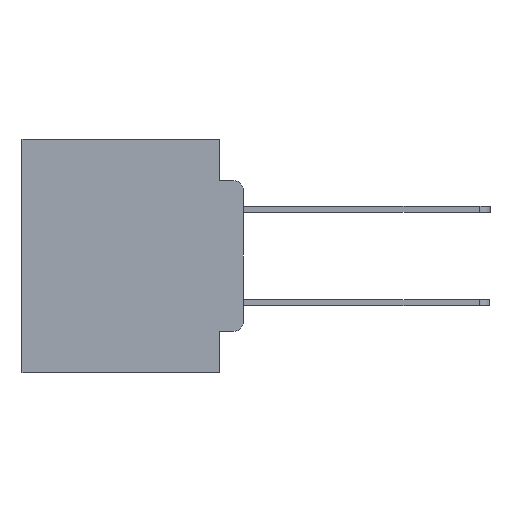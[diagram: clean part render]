
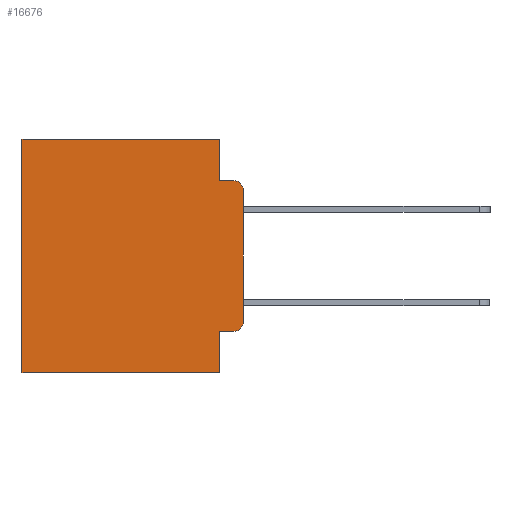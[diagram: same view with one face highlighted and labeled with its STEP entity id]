
A CAD part, left-side view. The second image highlights one B-rep face of the part: STEP entity #16676.
In plain terms, the highlighted planar face has unit normal (-1, 0, 0).
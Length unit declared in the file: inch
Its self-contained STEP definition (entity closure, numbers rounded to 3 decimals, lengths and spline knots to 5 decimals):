
#550 = LINE ( 'NONE', #1468, #6567 ) ;
#608 = VERTEX_POINT ( 'NONE', #22493 ) ;
#1370 = DIRECTION ( 'NONE',  ( 0., -1., 0. ) ) ;
#1468 = CARTESIAN_POINT ( 'NONE',  ( 0.298, 0.051, -0.0885 ) ) ;
#1498 = CARTESIAN_POINT ( 'NONE',  ( 0.298, 0., 0. ) ) ;
#1884 = ORIENTED_EDGE ( 'NONE', *, *, #14742, .F. ) ;
#2180 = VERTEX_POINT ( 'NONE', #12325 ) ;
#2238 = ORIENTED_EDGE ( 'NONE', *, *, #26624, .F. ) ;
#2448 = ORIENTED_EDGE ( 'NONE', *, *, #19890, .F. ) ;
#2474 = AXIS2_PLACEMENT_3D ( 'NONE', #1498, #10441, #24850 ) ;
#2882 = VECTOR ( 'NONE', #9533, 39.37008 ) ;
#3536 = CARTESIAN_POINT ( 'NONE',  ( 0.298, 0.051, -0.4115 ) ) ;
#3765 = CARTESIAN_POINT ( 'NONE',  ( 0.298, 0.473, 0. ) ) ;
#4331 = CARTESIAN_POINT ( 'NONE',  ( 0.298, 0.02, -0.1085 ) ) ;
#4355 = LINE ( 'NONE', #17075, #25990 ) ;
#4392 = CIRCLE ( 'NONE', #5933, 0.02 ) ;
#5150 = ORIENTED_EDGE ( 'NONE', *, *, #14354, .T. ) ;
#5281 = FACE_OUTER_BOUND ( 'NONE', #22569, .T. ) ;
#5768 = ORIENTED_EDGE ( 'NONE', *, *, #21215, .T. ) ;
#5933 = AXIS2_PLACEMENT_3D ( 'NONE', #4331, #19269, #6563 ) ;
#6232 = VERTEX_POINT ( 'NONE', #3765 ) ;
#6381 = DIRECTION ( 'NONE',  ( 0., 0., -1. ) ) ;
#6542 = VERTEX_POINT ( 'NONE', #9163 ) ;
#6563 = DIRECTION ( 'NONE',  ( 0., 0., -1. ) ) ;
#6567 = VECTOR ( 'NONE', #1370, 39.37008 ) ;
#6647 = EDGE_CURVE ( 'NONE', #6232, #12560, #23964, .T. ) ;
#7183 = EDGE_CURVE ( 'NONE', #18564, #608, #27380, .T. ) ;
#7649 = VERTEX_POINT ( 'NONE', #26843 ) ;
#8199 = VECTOR ( 'NONE', #15817, 39.37008 ) ;
#8276 = LINE ( 'NONE', #17052, #18820 ) ;
#9163 = CARTESIAN_POINT ( 'NONE',  ( 0.298, 0.051, -0.5 ) ) ;
#9533 = DIRECTION ( 'NONE',  ( 0., 0., -1. ) ) ;
#9902 = DIRECTION ( 'NONE',  ( -1., 0., 0. ) ) ;
#10441 = DIRECTION ( 'NONE',  ( 1., 0., 0. ) ) ;
#10773 = CARTESIAN_POINT ( 'NONE',  ( 0.298, 0.02, -0.0885 ) ) ;
#11007 = DIRECTION ( 'NONE',  ( 0., 0., -1. ) ) ;
#11294 = CARTESIAN_POINT ( 'NONE',  ( 0.298, 0.051, -0.4115 ) ) ;
#12325 = CARTESIAN_POINT ( 'NONE',  ( 0.298, 0.051, -0.0885 ) ) ;
#12560 = VERTEX_POINT ( 'NONE', #13832 ) ;
#13065 = VERTEX_POINT ( 'NONE', #17777 ) ;
#13832 = CARTESIAN_POINT ( 'NONE',  ( 0.298, 0.473, -0.5 ) ) ;
#13843 = CARTESIAN_POINT ( 'NONE',  ( 0.298, 0., 0. ) ) ;
#13853 = LINE ( 'NONE', #13843, #2882 ) ;
#14046 = ORIENTED_EDGE ( 'NONE', *, *, #19432, .F. ) ;
#14354 = EDGE_CURVE ( 'NONE', #13065, #6232, #14584, .T. ) ;
#14584 = LINE ( 'NONE', #25925, #8199 ) ;
#14742 = EDGE_CURVE ( 'NONE', #6542, #12560, #4355, .T. ) ;
#15424 = DIRECTION ( 'NONE',  ( 0., -1., 0. ) ) ;
#15817 = DIRECTION ( 'NONE',  ( 0., 1., 0. ) ) ;
#15904 = DIRECTION ( 'NONE',  ( 0., 0., -1. ) ) ;
#16362 = VERTEX_POINT ( 'NONE', #17791 ) ;
#16676 = ADVANCED_FACE ( 'NONE', ( #5281 ), #18743, .F. ) ;
#17052 = CARTESIAN_POINT ( 'NONE',  ( 0.298, 0.051, 0. ) ) ;
#17075 = CARTESIAN_POINT ( 'NONE',  ( 0.298, 0., -0.5 ) ) ;
#17703 = EDGE_CURVE ( 'NONE', #608, #16362, #23693, .T. ) ;
#17777 = CARTESIAN_POINT ( 'NONE',  ( 0.298, 0.051, 0. ) ) ;
#17791 = CARTESIAN_POINT ( 'NONE',  ( 0.298, 0., -0.3915 ) ) ;
#17918 = VECTOR ( 'NONE', #11007, 39.37008 ) ;
#18536 = LINE ( 'NONE', #27291, #17918 ) ;
#18564 = VERTEX_POINT ( 'NONE', #3536 ) ;
#18571 = VECTOR ( 'NONE', #15904, 39.37008 ) ;
#18743 = PLANE ( 'NONE',  #2474 ) ;
#18820 = VECTOR ( 'NONE', #6381, 39.37008 ) ;
#19269 = DIRECTION ( 'NONE',  ( -1., 0., 0. ) ) ;
#19432 = EDGE_CURVE ( 'NONE', #13065, #2180, #18536, .T. ) ;
#19890 = EDGE_CURVE ( 'NONE', #2180, #23614, #550, .T. ) ;
#19932 = CARTESIAN_POINT ( 'NONE',  ( 0.298, 0.473, 0. ) ) ;
#19948 = ORIENTED_EDGE ( 'NONE', *, *, #23970, .F. ) ;
#19999 = ORIENTED_EDGE ( 'NONE', *, *, #6647, .T. ) ;
#21066 = ORIENTED_EDGE ( 'NONE', *, *, #17703, .T. ) ;
#21215 = EDGE_CURVE ( 'NONE', #7649, #23614, #4392, .T. ) ;
#22289 = CARTESIAN_POINT ( 'NONE',  ( 0.298, 0.02, -0.3915 ) ) ;
#22493 = CARTESIAN_POINT ( 'NONE',  ( 0.298, 0.02, -0.4115 ) ) ;
#22569 = EDGE_LOOP ( 'NONE', ( #2238, #5768, #2448, #14046, #5150, #19999, #1884, #19948, #23848, #21066 ) ) ;
#23614 = VERTEX_POINT ( 'NONE', #10773 ) ;
#23693 = CIRCLE ( 'NONE', #26657, 0.02 ) ;
#23848 = ORIENTED_EDGE ( 'NONE', *, *, #7183, .T. ) ;
#23964 = LINE ( 'NONE', #19932, #18571 ) ;
#23970 = EDGE_CURVE ( 'NONE', #18564, #6542, #8276, .T. ) ;
#24348 = DIRECTION ( 'NONE',  ( 0., 0., -1. ) ) ;
#24850 = DIRECTION ( 'NONE',  ( 0., 0., -1. ) ) ;
#25297 = DIRECTION ( 'NONE',  ( 0., 1., 0. ) ) ;
#25925 = CARTESIAN_POINT ( 'NONE',  ( 0.298, 0., 0. ) ) ;
#25990 = VECTOR ( 'NONE', #25297, 39.37008 ) ;
#26624 = EDGE_CURVE ( 'NONE', #7649, #16362, #13853, .T. ) ;
#26657 = AXIS2_PLACEMENT_3D ( 'NONE', #22289, #9902, #24348 ) ;
#26767 = VECTOR ( 'NONE', #15424, 39.37008 ) ;
#26843 = CARTESIAN_POINT ( 'NONE',  ( 0.298, 0., -0.1085 ) ) ;
#27291 = CARTESIAN_POINT ( 'NONE',  ( 0.298, 0.051, 0. ) ) ;
#27380 = LINE ( 'NONE', #11294, #26767 ) ;
